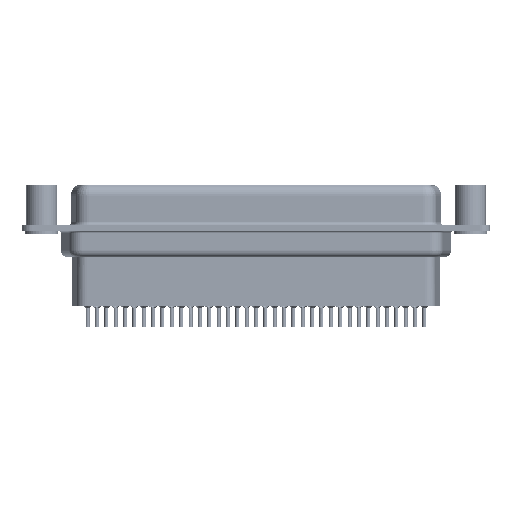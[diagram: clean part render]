
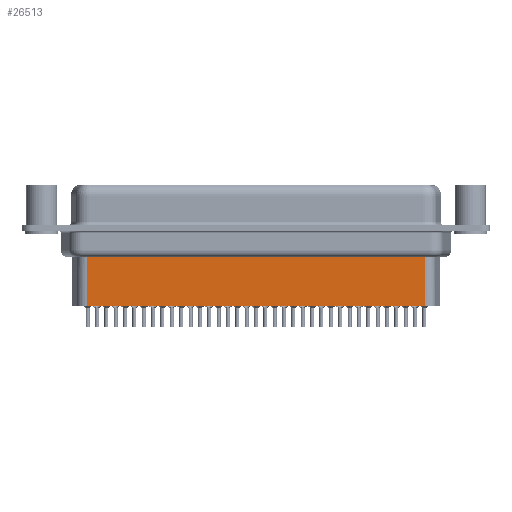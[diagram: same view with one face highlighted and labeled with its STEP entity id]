
A CAD part, front view. The second image highlights one B-rep face of the part: STEP entity #26513.
In plain terms, the highlighted planar face has unit normal (0, -1, 0).
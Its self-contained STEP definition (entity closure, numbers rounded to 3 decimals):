
#1734 = AXIS2_PLACEMENT_3D ( 'NONE', #26927, #21999, #6904 ) ;
#1836 = CARTESIAN_POINT ( 'NONE',  ( 56.794, -3.5, -11.45 ) ) ;
#3206 = EDGE_CURVE ( 'NONE', #7808, #15130, #4079, .T. ) ;
#3817 = ORIENTED_EDGE ( 'NONE', *, *, #8787, .T. ) ;
#4079 = LINE ( 'NONE', #5969, #15308 ) ;
#5969 = CARTESIAN_POINT ( 'NONE',  ( 6.459, -3.5, -4.097 ) ) ;
#5977 = DIRECTION ( 'NONE',  ( -1., 0., 0. ) ) ;
#6904 = DIRECTION ( 'NONE',  ( 1., 0., 0. ) ) ;
#7162 = CARTESIAN_POINT ( 'NONE',  ( 6.706, -3.5, -4.097 ) ) ;
#7808 = VERTEX_POINT ( 'NONE', #26590 ) ;
#8314 = VECTOR ( 'NONE', #30210, 1000. ) ;
#8698 = ORIENTED_EDGE ( 'NONE', *, *, #3206, .T. ) ;
#8787 = EDGE_CURVE ( 'NONE', #15130, #13807, #13530, .T. ) ;
#8848 = EDGE_LOOP ( 'NONE', ( #28864, #8698, #3817, #25929 ) ) ;
#12655 = DIRECTION ( 'NONE',  ( 0., 0., -1. ) ) ;
#12865 = EDGE_CURVE ( 'NONE', #7808, #24246, #20354, .T. ) ;
#13530 = LINE ( 'NONE', #32711, #8314 ) ;
#13807 = VERTEX_POINT ( 'NONE', #14142 ) ;
#14142 = CARTESIAN_POINT ( 'NONE',  ( 6.706, -3.5, -11.45 ) ) ;
#15130 = VERTEX_POINT ( 'NONE', #7162 ) ;
#15308 = VECTOR ( 'NONE', #5977, 1000. ) ;
#16953 = CARTESIAN_POINT ( 'NONE',  ( 6.706, -3.5, -11.45 ) ) ;
#18607 = VECTOR ( 'NONE', #27040, 1000. ) ;
#19505 = PLANE ( 'NONE',  #1734 ) ;
#20354 = LINE ( 'NONE', #27596, #26228 ) ;
#21999 = DIRECTION ( 'NONE',  ( 0., -1., 0. ) ) ;
#24246 = VERTEX_POINT ( 'NONE', #1836 ) ;
#25239 = LINE ( 'NONE', #16953, #18607 ) ;
#25929 = ORIENTED_EDGE ( 'NONE', *, *, #30184, .F. ) ;
#25940 = FACE_OUTER_BOUND ( 'NONE', #8848, .T. ) ;
#26228 = VECTOR ( 'NONE', #12655, 1000. ) ;
#26513 = ADVANCED_FACE ( 'NONE', ( #25940 ), #19505, .T. ) ;
#26590 = CARTESIAN_POINT ( 'NONE',  ( 56.794, -3.5, -4.097 ) ) ;
#26927 = CARTESIAN_POINT ( 'NONE',  ( 6.706, -3.5, -3.1 ) ) ;
#27040 = DIRECTION ( 'NONE',  ( -1., 0., 0. ) ) ;
#27596 = CARTESIAN_POINT ( 'NONE',  ( 56.794, -3.5, -3.1 ) ) ;
#28864 = ORIENTED_EDGE ( 'NONE', *, *, #12865, .F. ) ;
#30184 = EDGE_CURVE ( 'NONE', #24246, #13807, #25239, .T. ) ;
#30210 = DIRECTION ( 'NONE',  ( 0., 0., -1. ) ) ;
#32711 = CARTESIAN_POINT ( 'NONE',  ( 6.706, -3.5, -3.1 ) ) ;
